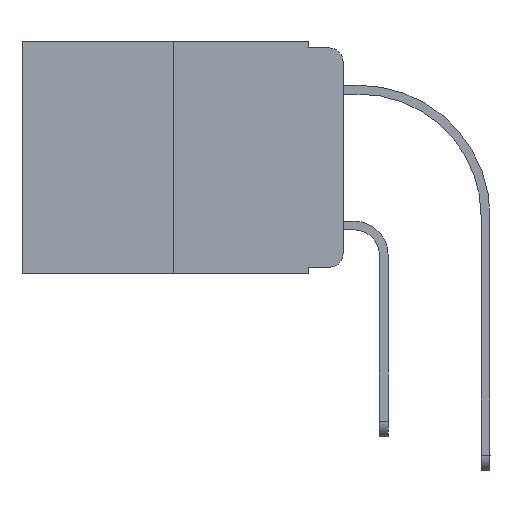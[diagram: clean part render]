
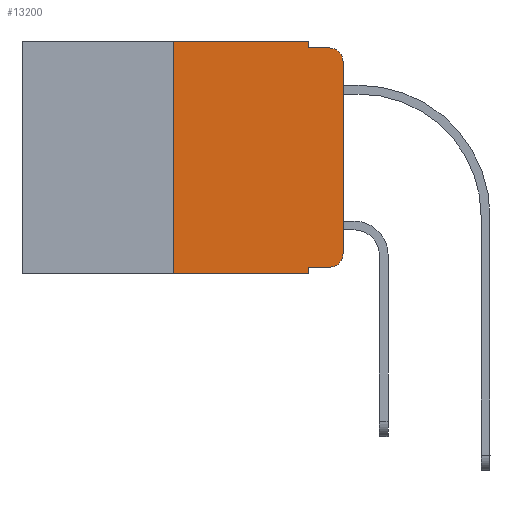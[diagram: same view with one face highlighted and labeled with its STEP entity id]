
A CAD part, left-side view. The second image highlights one B-rep face of the part: STEP entity #13200.
In plain terms, the highlighted planar face has unit normal (-1, 0, 0).
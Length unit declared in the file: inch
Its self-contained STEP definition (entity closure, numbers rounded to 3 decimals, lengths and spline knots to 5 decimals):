
#234 = VERTEX_POINT ( 'NONE', #7646 ) ;
#281 = VECTOR ( 'NONE', #813, 39.37008 ) ;
#461 = DIRECTION ( 'NONE',  ( -1., 0., 0. ) ) ;
#713 = CARTESIAN_POINT ( 'NONE',  ( 0., 0.02, -0.313 ) ) ;
#784 = CARTESIAN_POINT ( 'NONE',  ( 0., 0.02, -0.01 ) ) ;
#813 = DIRECTION ( 'NONE',  ( 0., 0., -1. ) ) ;
#1112 = CARTESIAN_POINT ( 'NONE',  ( 0., 0.051, -0.01 ) ) ;
#1138 = CARTESIAN_POINT ( 'NONE',  ( 0., 0.051, 0. ) ) ;
#1151 = ORIENTED_EDGE ( 'NONE', *, *, #3108, .F. ) ;
#1893 = LINE ( 'NONE', #1138, #281 ) ;
#2696 = FACE_OUTER_BOUND ( 'NONE', #4930, .T. ) ;
#2770 = PLANE ( 'NONE',  #12534 ) ;
#2772 = LINE ( 'NONE', #7193, #6880 ) ;
#3069 = CARTESIAN_POINT ( 'NONE',  ( 0., 0.051, -0.343 ) ) ;
#3101 = CARTESIAN_POINT ( 'NONE',  ( 0., 0., -0.313 ) ) ;
#3108 = EDGE_CURVE ( 'NONE', #3467, #6885, #13171, .T. ) ;
#3245 = CARTESIAN_POINT ( 'NONE',  ( 0., 0.051, 0. ) ) ;
#3264 = AXIS2_PLACEMENT_3D ( 'NONE', #12400, #461, #12333 ) ;
#3330 = DIRECTION ( 'NONE',  ( 0., 0., 1. ) ) ;
#3416 = VECTOR ( 'NONE', #11003, 39.37008 ) ;
#3428 = ORIENTED_EDGE ( 'NONE', *, *, #4841, .F. ) ;
#3445 = CARTESIAN_POINT ( 'NONE',  ( 0., 0.051, 0. ) ) ;
#3467 = VERTEX_POINT ( 'NONE', #3445 ) ;
#3509 = VECTOR ( 'NONE', #7951, 39.37008 ) ;
#4839 = EDGE_CURVE ( 'NONE', #6885, #11131, #11039, .T. ) ;
#4841 = EDGE_CURVE ( 'NONE', #12338, #8000, #1893, .T. ) ;
#4930 = EDGE_LOOP ( 'NONE', ( #12844, #8162, #9779, #1151, #9282, #9918, #6772, #3428, #8340, #11289 ) ) ;
#5002 = DIRECTION ( 'NONE',  ( 0., -1., 0. ) ) ;
#5474 = VECTOR ( 'NONE', #6260, 39.37008 ) ;
#5501 = CARTESIAN_POINT ( 'NONE',  ( 0., 0., 0. ) ) ;
#5876 = LINE ( 'NONE', #9422, #12447 ) ;
#6089 = VERTEX_POINT ( 'NONE', #9958 ) ;
#6260 = DIRECTION ( 'NONE',  ( 0., -1., 0. ) ) ;
#6772 = ORIENTED_EDGE ( 'NONE', *, *, #11493, .T. ) ;
#6880 = VECTOR ( 'NONE', #5002, 39.37008 ) ;
#6885 = VERTEX_POINT ( 'NONE', #1112 ) ;
#7010 = EDGE_CURVE ( 'NONE', #12338, #8766, #5876, .T. ) ;
#7120 = CARTESIAN_POINT ( 'NONE',  ( 0., 0.473, 0. ) ) ;
#7190 = DIRECTION ( 'NONE',  ( 0., 0., -1. ) ) ;
#7193 = CARTESIAN_POINT ( 'NONE',  ( 0., 0.473, 0. ) ) ;
#7357 = CARTESIAN_POINT ( 'NONE',  ( 0., 0., -0.03 ) ) ;
#7646 = CARTESIAN_POINT ( 'NONE',  ( 0., 0.25, 0. ) ) ;
#7951 = DIRECTION ( 'NONE',  ( 0., -1., 0. ) ) ;
#8000 = VERTEX_POINT ( 'NONE', #3069 ) ;
#8162 = ORIENTED_EDGE ( 'NONE', *, *, #14055, .T. ) ;
#8242 = DIRECTION ( 'NONE',  ( -1., 0., 0. ) ) ;
#8340 = ORIENTED_EDGE ( 'NONE', *, *, #7010, .T. ) ;
#8353 = EDGE_CURVE ( 'NONE', #234, #3467, #2772, .T. ) ;
#8766 = VERTEX_POINT ( 'NONE', #10480 ) ;
#8777 = CARTESIAN_POINT ( 'NONE',  ( 0., 0.25, 0. ) ) ;
#9235 = CARTESIAN_POINT ( 'NONE',  ( 0., 0.051, -0.333 ) ) ;
#9273 = DIRECTION ( 'NONE',  ( 0., -1., 0. ) ) ;
#9282 = ORIENTED_EDGE ( 'NONE', *, *, #8353, .F. ) ;
#9384 = DIRECTION ( 'NONE',  ( 0., 0., -1. ) ) ;
#9405 = VECTOR ( 'NONE', #3330, 39.37008 ) ;
#9422 = CARTESIAN_POINT ( 'NONE',  ( 0., 0.051, -0.333 ) ) ;
#9779 = ORIENTED_EDGE ( 'NONE', *, *, #4839, .F. ) ;
#9811 = EDGE_CURVE ( 'NONE', #6089, #234, #10730, .T. ) ;
#9918 = ORIENTED_EDGE ( 'NONE', *, *, #9811, .F. ) ;
#9958 = CARTESIAN_POINT ( 'NONE',  ( 0., 0.25, -0.343 ) ) ;
#9959 = CIRCLE ( 'NONE', #3264, 0.02 ) ;
#10480 = CARTESIAN_POINT ( 'NONE',  ( 0., 0.02, -0.333 ) ) ;
#10730 = LINE ( 'NONE', #8777, #3416 ) ;
#10954 = AXIS2_PLACEMENT_3D ( 'NONE', #713, #8242, #9384 ) ;
#10985 = VECTOR ( 'NONE', #12087, 39.37008 ) ;
#10988 = LINE ( 'NONE', #5501, #9405 ) ;
#11003 = DIRECTION ( 'NONE',  ( 0., 0., 1. ) ) ;
#11039 = LINE ( 'NONE', #12972, #3509 ) ;
#11131 = VERTEX_POINT ( 'NONE', #784 ) ;
#11289 = ORIENTED_EDGE ( 'NONE', *, *, #12249, .T. ) ;
#11493 = EDGE_CURVE ( 'NONE', #6089, #8000, #13869, .T. ) ;
#11520 = DIRECTION ( 'NONE',  ( 1., 0., 0. ) ) ;
#11583 = EDGE_CURVE ( 'NONE', #11945, #12793, #10988, .T. ) ;
#11945 = VERTEX_POINT ( 'NONE', #3101 ) ;
#12087 = DIRECTION ( 'NONE',  ( 0., 0., -1. ) ) ;
#12249 = EDGE_CURVE ( 'NONE', #8766, #11945, #12372, .T. ) ;
#12333 = DIRECTION ( 'NONE',  ( 0., 0., -1. ) ) ;
#12338 = VERTEX_POINT ( 'NONE', #9235 ) ;
#12372 = CIRCLE ( 'NONE', #10954, 0.02 ) ;
#12400 = CARTESIAN_POINT ( 'NONE',  ( 0., 0.02, -0.03 ) ) ;
#12447 = VECTOR ( 'NONE', #9273, 39.37008 ) ;
#12534 = AXIS2_PLACEMENT_3D ( 'NONE', #7120, #11520, #7190 ) ;
#12793 = VERTEX_POINT ( 'NONE', #7357 ) ;
#12844 = ORIENTED_EDGE ( 'NONE', *, *, #11583, .T. ) ;
#12972 = CARTESIAN_POINT ( 'NONE',  ( 0., 0.051, -0.01 ) ) ;
#13112 = CARTESIAN_POINT ( 'NONE',  ( 0., 0.473, -0.343 ) ) ;
#13171 = LINE ( 'NONE', #3245, #10985 ) ;
#13200 = ADVANCED_FACE ( 'NONE', ( #2696 ), #2770, .F. ) ;
#13869 = LINE ( 'NONE', #13112, #5474 ) ;
#14055 = EDGE_CURVE ( 'NONE', #12793, #11131, #9959, .T. ) ;
